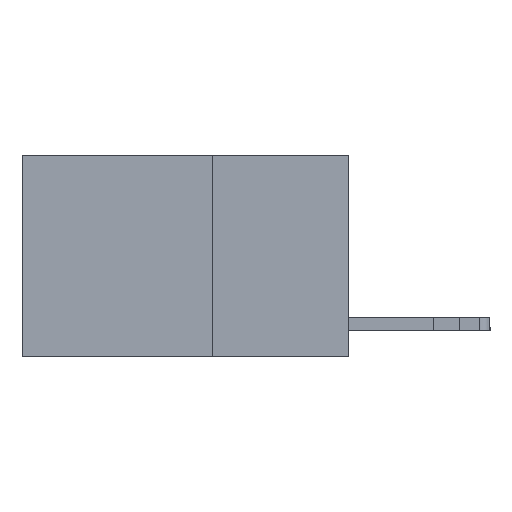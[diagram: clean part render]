
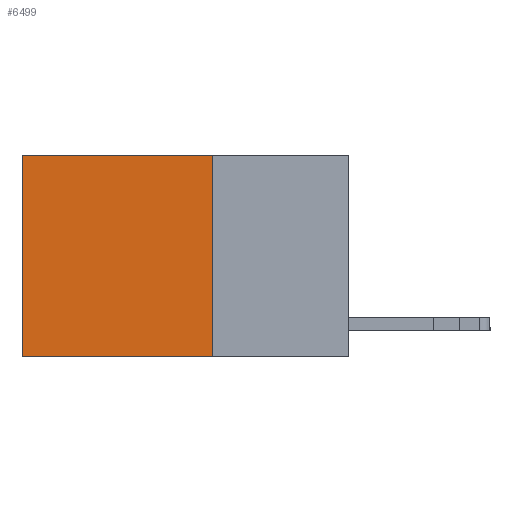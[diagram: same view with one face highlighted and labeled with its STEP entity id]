
A CAD part, left-side view. The second image highlights one B-rep face of the part: STEP entity #6499.
In plain terms, the highlighted planar face has unit normal (-1, 0, 0).
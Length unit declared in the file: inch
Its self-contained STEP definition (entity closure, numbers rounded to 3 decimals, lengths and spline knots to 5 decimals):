
#445 = LINE ( 'NONE', #5618, #11124 ) ;
#540 = CARTESIAN_POINT ( 'NONE',  ( 0.2625, 0.25, -0.37 ) ) ;
#684 = ORIENTED_EDGE ( 'NONE', *, *, #5250, .F. ) ;
#1483 = VECTOR ( 'NONE', #4794, 39.37008 ) ;
#1678 = CARTESIAN_POINT ( 'NONE',  ( 0.2625, 0.6, -0.37 ) ) ;
#2599 = CARTESIAN_POINT ( 'NONE',  ( 0.2625, 0.6, 0. ) ) ;
#3007 = EDGE_CURVE ( 'NONE', #3555, #3768, #15842, .T. ) ;
#3173 = VERTEX_POINT ( 'NONE', #11174 ) ;
#3464 = EDGE_CURVE ( 'NONE', #13391, #3768, #13454, .T. ) ;
#3555 = VERTEX_POINT ( 'NONE', #6983 ) ;
#3680 = DIRECTION ( 'NONE',  ( 0., 0., -1. ) ) ;
#3768 = VERTEX_POINT ( 'NONE', #1678 ) ;
#3956 = ORIENTED_EDGE ( 'NONE', *, *, #3464, .F. ) ;
#4343 = VECTOR ( 'NONE', #9619, 39.37008 ) ;
#4489 = ORIENTED_EDGE ( 'NONE', *, *, #3007, .T. ) ;
#4794 = DIRECTION ( 'NONE',  ( 0., 1., 0. ) ) ;
#5118 = PLANE ( 'NONE',  #16030 ) ;
#5137 = VECTOR ( 'NONE', #7773, 39.37008 ) ;
#5250 = EDGE_CURVE ( 'NONE', #3173, #13391, #445, .T. ) ;
#5618 = CARTESIAN_POINT ( 'NONE',  ( 0.2625, 0.25, 0. ) ) ;
#5639 = CARTESIAN_POINT ( 'NONE',  ( 0.2625, 0.25, -0.37 ) ) ;
#6499 = ADVANCED_FACE ( 'NONE', ( #13957 ), #5118, .F. ) ;
#6983 = CARTESIAN_POINT ( 'NONE',  ( 0.2625, 0.6, 0. ) ) ;
#7742 = DIRECTION ( 'NONE',  ( 1., 0., 0. ) ) ;
#7773 = DIRECTION ( 'NONE',  ( 0., 0., -1. ) ) ;
#9518 = DIRECTION ( 'NONE',  ( 0., 0., -1. ) ) ;
#9619 = DIRECTION ( 'NONE',  ( 0., 1., 0. ) ) ;
#10551 = EDGE_CURVE ( 'NONE', #3173, #3555, #12769, .T. ) ;
#11124 = VECTOR ( 'NONE', #9518, 39.37008 ) ;
#11174 = CARTESIAN_POINT ( 'NONE',  ( 0.2625, 0.25, 0. ) ) ;
#12769 = LINE ( 'NONE', #15226, #1483 ) ;
#13391 = VERTEX_POINT ( 'NONE', #540 ) ;
#13454 = LINE ( 'NONE', #5639, #4343 ) ;
#13957 = FACE_OUTER_BOUND ( 'NONE', #15908, .T. ) ;
#15226 = CARTESIAN_POINT ( 'NONE',  ( 0.2625, 0.25, 0. ) ) ;
#15498 = ORIENTED_EDGE ( 'NONE', *, *, #10551, .T. ) ;
#15842 = LINE ( 'NONE', #2599, #5137 ) ;
#15908 = EDGE_LOOP ( 'NONE', ( #4489, #3956, #684, #15498 ) ) ;
#16030 = AXIS2_PLACEMENT_3D ( 'NONE', #16665, #7742, #3680 ) ;
#16665 = CARTESIAN_POINT ( 'NONE',  ( 0.2625, 0.25, 0. ) ) ;
